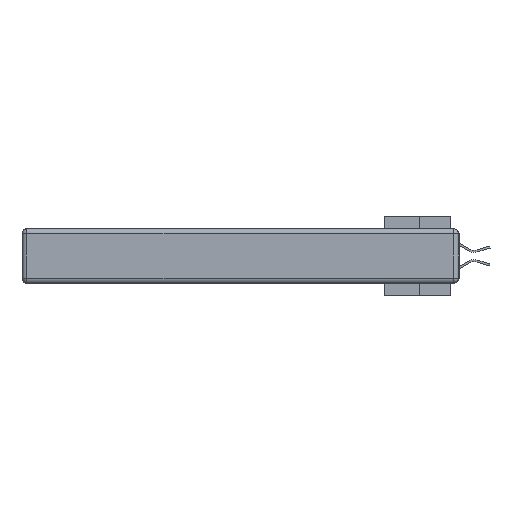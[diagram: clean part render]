
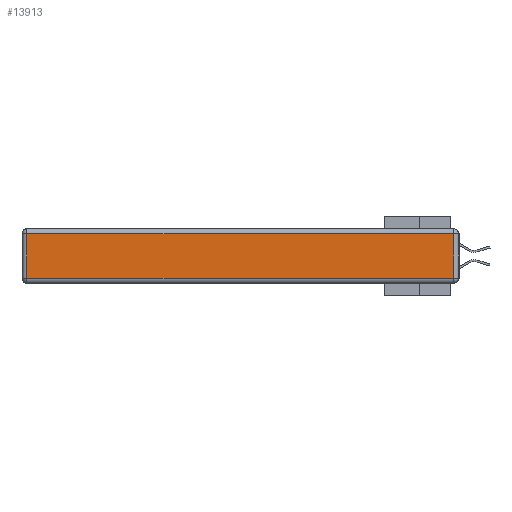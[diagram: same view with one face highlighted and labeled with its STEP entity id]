
A CAD part, left-side view. The second image highlights one B-rep face of the part: STEP entity #13913.
In plain terms, the highlighted planar face has unit normal (-1, 0, 0).
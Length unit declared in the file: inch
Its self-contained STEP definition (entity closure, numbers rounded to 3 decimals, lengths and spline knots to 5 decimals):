
#165 = DIRECTION ( 'NONE',  ( 0., 1., 0. ) ) ;
#1367 = VERTEX_POINT ( 'NONE', #16236 ) ;
#1447 = DIRECTION ( 'NONE',  ( 0., 0., 1. ) ) ;
#3675 = VERTEX_POINT ( 'NONE', #11348 ) ;
#4954 = ORIENTED_EDGE ( 'NONE', *, *, #24027, .T. ) ;
#7449 = CARTESIAN_POINT ( 'NONE',  ( 0., 2.72, -0.343 ) ) ;
#7811 = CARTESIAN_POINT ( 'NONE',  ( 0., 0., -0.313 ) ) ;
#8326 = VECTOR ( 'NONE', #1447, 39.37008 ) ;
#10099 = LINE ( 'NONE', #31197, #8326 ) ;
#10747 = ORIENTED_EDGE ( 'NONE', *, *, #15045, .T. ) ;
#10867 = DIRECTION ( 'NONE',  ( 0., -1., 0. ) ) ;
#10879 = LINE ( 'NONE', #7449, #23037 ) ;
#11074 = DIRECTION ( 'NONE',  ( 0., 0., -1. ) ) ;
#11205 = CARTESIAN_POINT ( 'NONE',  ( 0., 0.03, -0.313 ) ) ;
#11348 = CARTESIAN_POINT ( 'NONE',  ( 0., 2.72, -0.03 ) ) ;
#11619 = PLANE ( 'NONE',  #34466 ) ;
#13913 = ADVANCED_FACE ( 'NONE', ( #31968 ), #11619, .T. ) ;
#14671 = CARTESIAN_POINT ( 'NONE',  ( 0., 0., -0.343 ) ) ;
#15045 = EDGE_CURVE ( 'NONE', #1367, #25673, #34507, .T. ) ;
#15709 = ORIENTED_EDGE ( 'NONE', *, *, #19458, .T. ) ;
#16236 = CARTESIAN_POINT ( 'NONE',  ( 0., 2.72, -0.313 ) ) ;
#17548 = DIRECTION ( 'NONE',  ( 0., 0., 1. ) ) ;
#17640 = LINE ( 'NONE', #29352, #35701 ) ;
#19458 = EDGE_CURVE ( 'NONE', #25673, #22278, #10099, .T. ) ;
#22278 = VERTEX_POINT ( 'NONE', #34804 ) ;
#23037 = VECTOR ( 'NONE', #11074, 39.37008 ) ;
#24027 = EDGE_CURVE ( 'NONE', #22278, #3675, #17640, .T. ) ;
#25673 = VERTEX_POINT ( 'NONE', #11205 ) ;
#26192 = DIRECTION ( 'NONE',  ( -1., 0., 0. ) ) ;
#27653 = EDGE_LOOP ( 'NONE', ( #10747, #15709, #4954, #27968 ) ) ;
#27968 = ORIENTED_EDGE ( 'NONE', *, *, #28379, .T. ) ;
#28379 = EDGE_CURVE ( 'NONE', #3675, #1367, #10879, .T. ) ;
#29352 = CARTESIAN_POINT ( 'NONE',  ( 0., 2.75, -0.03 ) ) ;
#31197 = CARTESIAN_POINT ( 'NONE',  ( 0., 0.03, -0.343 ) ) ;
#31968 = FACE_OUTER_BOUND ( 'NONE', #27653, .T. ) ;
#32027 = VECTOR ( 'NONE', #10867, 39.37008 ) ;
#34466 = AXIS2_PLACEMENT_3D ( 'NONE', #14671, #26192, #17548 ) ;
#34507 = LINE ( 'NONE', #7811, #32027 ) ;
#34804 = CARTESIAN_POINT ( 'NONE',  ( 0., 0.03, -0.03 ) ) ;
#35701 = VECTOR ( 'NONE', #165, 39.37008 ) ;
